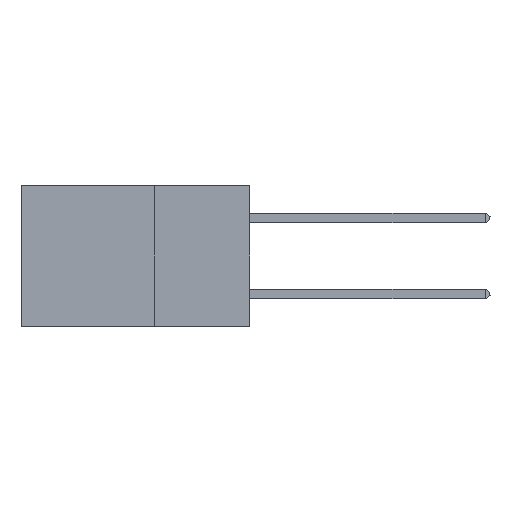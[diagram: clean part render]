
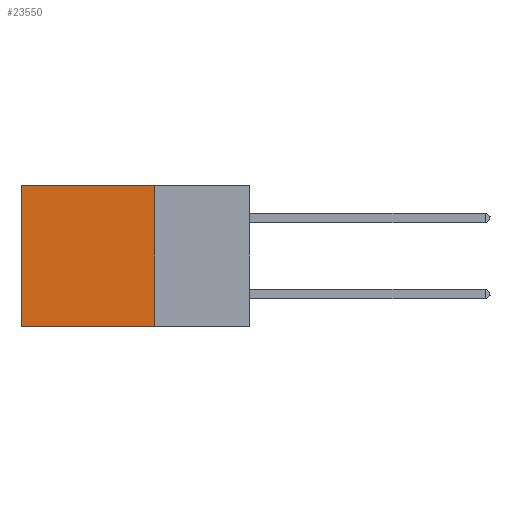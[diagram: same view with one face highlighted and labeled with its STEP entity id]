
A CAD part, left-side view. The second image highlights one B-rep face of the part: STEP entity #23550.
In plain terms, the highlighted planar face has unit normal (-1, 0, 0).
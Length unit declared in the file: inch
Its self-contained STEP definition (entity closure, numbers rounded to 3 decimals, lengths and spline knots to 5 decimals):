
#1254 = ORIENTED_EDGE ( 'NONE', *, *, #26346, .F. ) ;
#2941 = CARTESIAN_POINT ( 'NONE',  ( 0.2875, 0.25, -0.37 ) ) ;
#4047 = LINE ( 'NONE', #14442, #20049 ) ;
#5219 = CARTESIAN_POINT ( 'NONE',  ( 0.2875, 0.25, -0.37 ) ) ;
#6047 = CARTESIAN_POINT ( 'NONE',  ( 0.2875, 0.6, 0. ) ) ;
#6113 = EDGE_LOOP ( 'NONE', ( #26357, #1254, #23160, #17476 ) ) ;
#7784 = VECTOR ( 'NONE', #31956, 39.37008 ) ;
#9272 = DIRECTION ( 'NONE',  ( 0., 0., -1. ) ) ;
#10878 = EDGE_CURVE ( 'NONE', #28166, #16996, #29605, .T. ) ;
#11927 = CARTESIAN_POINT ( 'NONE',  ( 0.2875, 0.25, 0. ) ) ;
#14442 = CARTESIAN_POINT ( 'NONE',  ( 0.2875, 0.6, 0. ) ) ;
#14531 = CARTESIAN_POINT ( 'NONE',  ( 0.2875, 0.25, 0. ) ) ;
#16996 = VERTEX_POINT ( 'NONE', #6047 ) ;
#16997 = CARTESIAN_POINT ( 'NONE',  ( 0.2875, 0.25, 0. ) ) ;
#17476 = ORIENTED_EDGE ( 'NONE', *, *, #10878, .T. ) ;
#19863 = DIRECTION ( 'NONE',  ( 1., 0., 0. ) ) ;
#20049 = VECTOR ( 'NONE', #9272, 39.37008 ) ;
#20074 = DIRECTION ( 'NONE',  ( 0., 1., 0. ) ) ;
#20534 = VERTEX_POINT ( 'NONE', #33397 ) ;
#23160 = ORIENTED_EDGE ( 'NONE', *, *, #24412, .F. ) ;
#23271 = VECTOR ( 'NONE', #27282, 39.37008 ) ;
#23550 = ADVANCED_FACE ( 'NONE', ( #35778 ), #34029, .F. ) ;
#24412 = EDGE_CURVE ( 'NONE', #28166, #30632, #30853, .T. ) ;
#25375 = EDGE_CURVE ( 'NONE', #16996, #20534, #4047, .T. ) ;
#26346 = EDGE_CURVE ( 'NONE', #30632, #20534, #30945, .T. ) ;
#26357 = ORIENTED_EDGE ( 'NONE', *, *, #25375, .T. ) ;
#27282 = DIRECTION ( 'NONE',  ( 0., 0., -1. ) ) ;
#28166 = VERTEX_POINT ( 'NONE', #14531 ) ;
#29605 = LINE ( 'NONE', #11927, #7784 ) ;
#30020 = AXIS2_PLACEMENT_3D ( 'NONE', #16997, #19863, #34282 ) ;
#30632 = VERTEX_POINT ( 'NONE', #5219 ) ;
#30853 = LINE ( 'NONE', #35461, #23271 ) ;
#30945 = LINE ( 'NONE', #2941, #32709 ) ;
#31956 = DIRECTION ( 'NONE',  ( 0., 1., 0. ) ) ;
#32709 = VECTOR ( 'NONE', #20074, 39.37008 ) ;
#33397 = CARTESIAN_POINT ( 'NONE',  ( 0.2875, 0.6, -0.37 ) ) ;
#34029 = PLANE ( 'NONE',  #30020 ) ;
#34282 = DIRECTION ( 'NONE',  ( 0., 0., -1. ) ) ;
#35461 = CARTESIAN_POINT ( 'NONE',  ( 0.2875, 0.25, 0. ) ) ;
#35778 = FACE_OUTER_BOUND ( 'NONE', #6113, .T. ) ;
